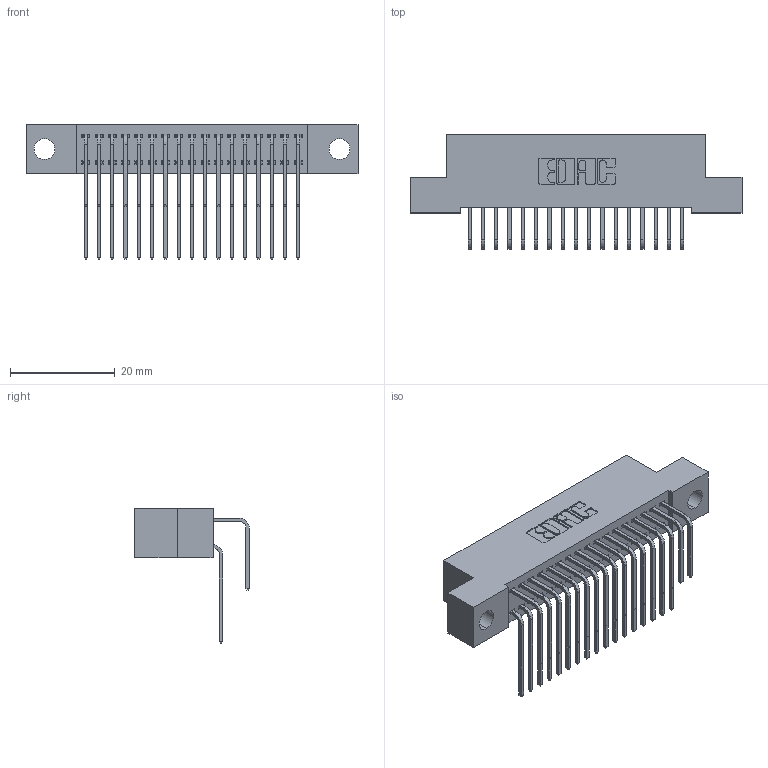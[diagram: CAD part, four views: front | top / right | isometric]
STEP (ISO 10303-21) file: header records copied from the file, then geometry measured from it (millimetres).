
FILE_DESCRIPTION (( 'STEP AP203' ), '1' );
FILE_NAME ('392-034-558-204.STEP', '2019-10-07T16:16:29', ( '' ), ( '' ), 'SwSTEP 2.0', 'SolidWorks 2016', '' );
FILE_SCHEMA (( 'CONFIG_CONTROL_DESIGN' ));
Length unit declared in the file: inch
Products named in the file (4): 342 Part_.156 TH; 345-292-001_558 559 Tail - 1; 345-292-001_558 Tail - 2; 392-034-558-204
Assembly tree (35 placements, depth 2):
  392-034-558-204
    342 Part_.156 TH
    345-292-001_558 559 Tail - 1  x17
    345-292-001_558 Tail - 2  x17
Bounding box: 63.5 x 21.91 x 25.78 mm (x, y, z)
Volume: 5696.2 mm3; surface area: 9367.5 mm2
Topology: 35 solids, 35 shells, 1946 faces, 5773 edges, 3802 vertices
Faces by surface type: plane 1358, cylinder 588
Entity records: 15825 total; most frequent: CARTESIAN_POINT 2701, ORIENTED_EDGE 2586, DIRECTION 2333, EDGE_CURVE 1293, LINE 1125, VECTOR 1125, VERTEX_POINT 858, AXIS2_PLACEMENT_3D 604
